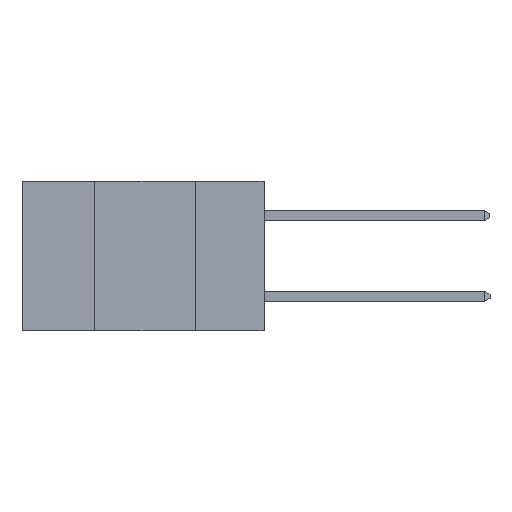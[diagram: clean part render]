
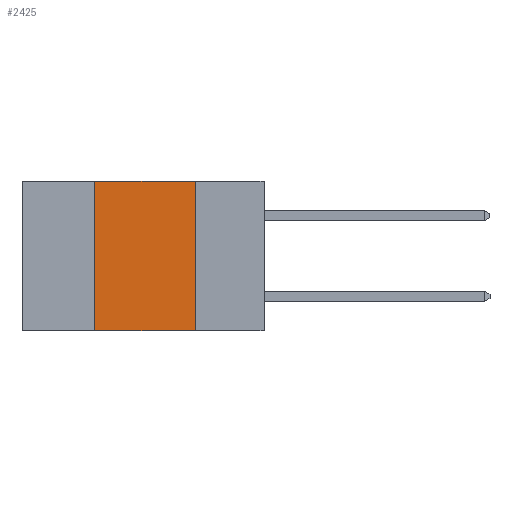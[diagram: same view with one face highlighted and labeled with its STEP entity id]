
A CAD part, left-side view. The second image highlights one B-rep face of the part: STEP entity #2425.
In plain terms, the highlighted planar face has unit normal (-1, 0, 0).
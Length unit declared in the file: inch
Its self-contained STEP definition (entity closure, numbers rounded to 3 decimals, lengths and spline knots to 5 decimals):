
#250 = EDGE_LOOP ( 'NONE', ( #7416, #8759, #5897, #3325 ) ) ;
#262 = AXIS2_PLACEMENT_3D ( 'NONE', #2387, #5317, #5246 ) ;
#486 = DIRECTION ( 'NONE',  ( 0., -1., 0. ) ) ;
#503 = EDGE_CURVE ( 'NONE', #4520, #1008, #691, .T. ) ;
#691 = LINE ( 'NONE', #4414, #8480 ) ;
#767 = PLANE ( 'NONE',  #262 ) ;
#970 = EDGE_CURVE ( 'NONE', #4153, #5518, #4770, .T. ) ;
#1008 = VERTEX_POINT ( 'NONE', #6369 ) ;
#1579 = VECTOR ( 'NONE', #1757, 39.37008 ) ;
#1757 = DIRECTION ( 'NONE',  ( 0., 0., -1. ) ) ;
#2345 = FACE_OUTER_BOUND ( 'NONE', #250, .T. ) ;
#2387 = CARTESIAN_POINT ( 'NONE',  ( 0., 0.6, 0. ) ) ;
#2425 = ADVANCED_FACE ( 'NONE', ( #2345 ), #767, .F. ) ;
#2687 = VECTOR ( 'NONE', #486, 39.37008 ) ;
#2760 = CARTESIAN_POINT ( 'NONE',  ( 0., 0.42, 0. ) ) ;
#3325 = ORIENTED_EDGE ( 'NONE', *, *, #970, .T. ) ;
#3398 = CARTESIAN_POINT ( 'NONE',  ( 0., 0.42, -0.37 ) ) ;
#3545 = LINE ( 'NONE', #4803, #1579 ) ;
#3666 = EDGE_CURVE ( 'NONE', #4153, #4520, #5306, .T. ) ;
#4153 = VERTEX_POINT ( 'NONE', #3398 ) ;
#4414 = CARTESIAN_POINT ( 'NONE',  ( 0., 0.6, 0. ) ) ;
#4520 = VERTEX_POINT ( 'NONE', #2760 ) ;
#4770 = LINE ( 'NONE', #5831, #2687 ) ;
#4803 = CARTESIAN_POINT ( 'NONE',  ( 0., 0.17, -0.37 ) ) ;
#5246 = DIRECTION ( 'NONE',  ( 0., 0., -1. ) ) ;
#5299 = CARTESIAN_POINT ( 'NONE',  ( 0., 0.42, -0.37 ) ) ;
#5306 = LINE ( 'NONE', #5299, #8968 ) ;
#5317 = DIRECTION ( 'NONE',  ( 1., 0., 0. ) ) ;
#5329 = DIRECTION ( 'NONE',  ( 0., 0., 1. ) ) ;
#5518 = VERTEX_POINT ( 'NONE', #9643 ) ;
#5730 = DIRECTION ( 'NONE',  ( 0., -1., 0. ) ) ;
#5831 = CARTESIAN_POINT ( 'NONE',  ( 0., 0.6, -0.37 ) ) ;
#5897 = ORIENTED_EDGE ( 'NONE', *, *, #3666, .F. ) ;
#6369 = CARTESIAN_POINT ( 'NONE',  ( 0., 0.17, 0. ) ) ;
#7416 = ORIENTED_EDGE ( 'NONE', *, *, #9588, .F. ) ;
#8480 = VECTOR ( 'NONE', #5730, 39.37008 ) ;
#8759 = ORIENTED_EDGE ( 'NONE', *, *, #503, .F. ) ;
#8968 = VECTOR ( 'NONE', #5329, 39.37008 ) ;
#9588 = EDGE_CURVE ( 'NONE', #1008, #5518, #3545, .T. ) ;
#9643 = CARTESIAN_POINT ( 'NONE',  ( 0., 0.17, -0.37 ) ) ;
